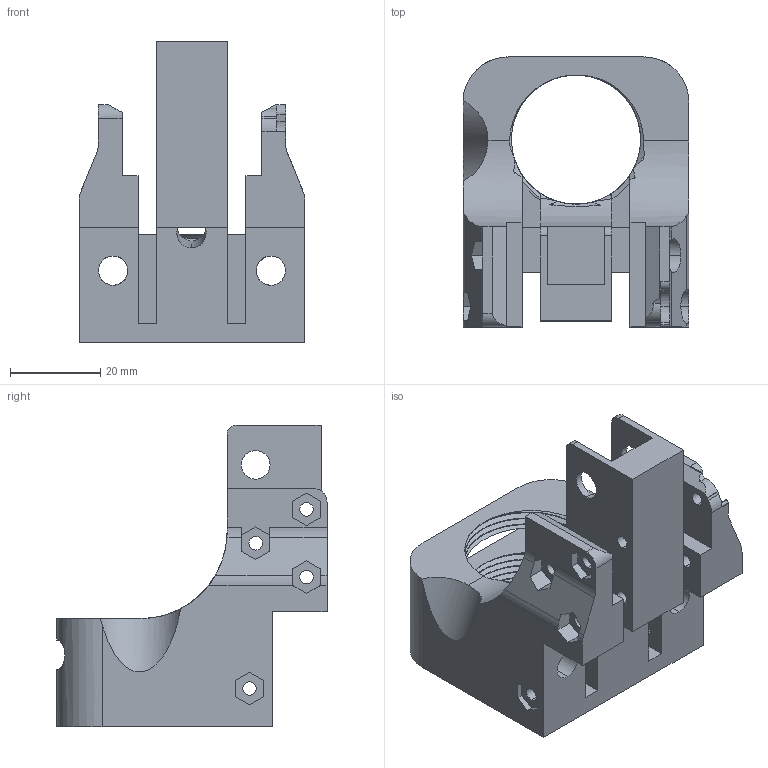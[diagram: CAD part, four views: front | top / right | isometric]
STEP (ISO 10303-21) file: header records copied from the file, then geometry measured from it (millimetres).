
FILE_DESCRIPTION (( 'STEP AP214' ), '1' );
FILE_NAME ('Thunderbolt_Buffer Tower_Split_Tower.STEP', '2021-09-21T22:19:51', ( '' ), ( '' ), 'SwSTEP 2.0', 'SolidWorks 2020', '' );
FILE_SCHEMA (( 'AUTOMOTIVE_DESIGN' ));
Length unit declared in the file: millimetre
Products named in the file (1): Thunderbolt_Buffer Tower_Split_Tower
Bounding box: 50 x 59.79 x 66.81 mm (x, y, z)
Volume: 55348 mm3; surface area: 23411.3 mm2
Topology: 1 solids, 1 shells, 234 faces, 699 edges, 463 vertices
Faces by surface type: cylinder 104, plane 88, bspline 38, cone 4
Entity records: 31311 total; most frequent: CARTESIAN_POINT 25495, ORIENTED_EDGE 1398, DIRECTION 980, EDGE_CURVE 699, VERTEX_POINT 463, AXIS2_PLACEMENT_3D 334, VECTOR 312, LINE 312
